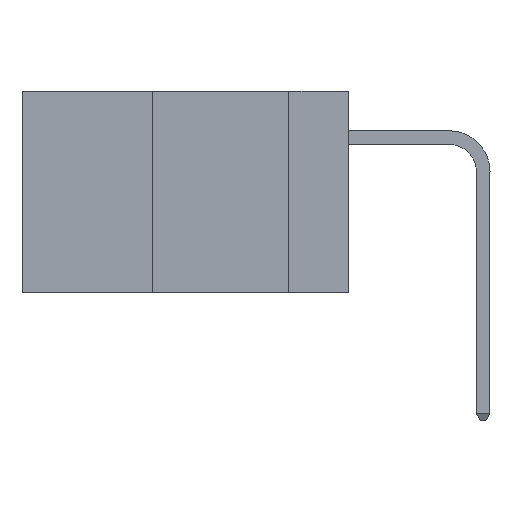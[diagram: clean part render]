
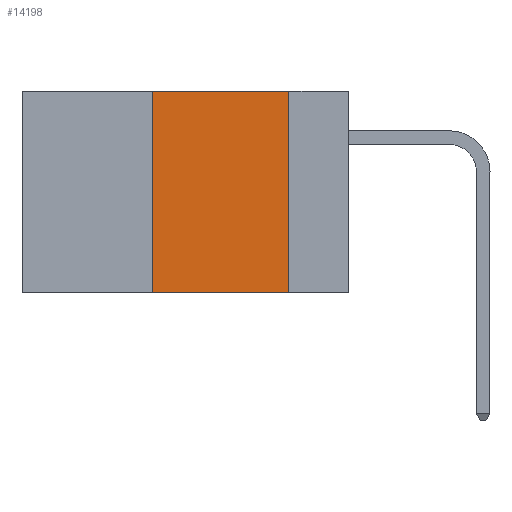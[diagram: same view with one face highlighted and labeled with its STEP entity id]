
A CAD part, left-side view. The second image highlights one B-rep face of the part: STEP entity #14198.
In plain terms, the highlighted planar face has unit normal (-1, 0, 0).
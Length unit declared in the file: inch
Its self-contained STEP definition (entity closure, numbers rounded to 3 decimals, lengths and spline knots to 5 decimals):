
#286 = LINE ( 'NONE', #26211, #30378 ) ;
#322 = ORIENTED_EDGE ( 'NONE', *, *, #28222, .F. ) ;
#530 = DIRECTION ( 'NONE',  ( 0., -1., 0. ) ) ;
#1850 = ORIENTED_EDGE ( 'NONE', *, *, #7102, .T. ) ;
#1885 = LINE ( 'NONE', #28804, #24264 ) ;
#4519 = EDGE_CURVE ( 'NONE', #36708, #11332, #286, .T. ) ;
#5098 = VECTOR ( 'NONE', #530, 39.37008 ) ;
#7102 = EDGE_CURVE ( 'NONE', #7261, #11332, #21603, .T. ) ;
#7261 = VERTEX_POINT ( 'NONE', #18776 ) ;
#9063 = PLANE ( 'NONE',  #30794 ) ;
#10246 = VERTEX_POINT ( 'NONE', #14431 ) ;
#11332 = VERTEX_POINT ( 'NONE', #33572 ) ;
#11418 = EDGE_LOOP ( 'NONE', ( #18640, #14074, #322, #1850 ) ) ;
#12031 = DIRECTION ( 'NONE',  ( 1., 0., 0. ) ) ;
#13965 = FACE_OUTER_BOUND ( 'NONE', #11418, .T. ) ;
#14074 = ORIENTED_EDGE ( 'NONE', *, *, #23675, .F. ) ;
#14198 = ADVANCED_FACE ( 'NONE', ( #13965 ), #9063, .F. ) ;
#14431 = CARTESIAN_POINT ( 'NONE',  ( 0., 0.36, 0. ) ) ;
#16020 = CARTESIAN_POINT ( 'NONE',  ( 0., 0.11, 0. ) ) ;
#18135 = CARTESIAN_POINT ( 'NONE',  ( 0., 0.6, -0.37 ) ) ;
#18640 = ORIENTED_EDGE ( 'NONE', *, *, #4519, .F. ) ;
#18776 = CARTESIAN_POINT ( 'NONE',  ( 0., 0.36, -0.37 ) ) ;
#20173 = VECTOR ( 'NONE', #25773, 39.37008 ) ;
#20572 = DIRECTION ( 'NONE',  ( 0., 0., -1. ) ) ;
#21603 = LINE ( 'NONE', #18135, #5098 ) ;
#22890 = CARTESIAN_POINT ( 'NONE',  ( 0., 0.6, 0. ) ) ;
#23675 = EDGE_CURVE ( 'NONE', #10246, #36708, #27820, .T. ) ;
#24264 = VECTOR ( 'NONE', #26007, 39.37008 ) ;
#25773 = DIRECTION ( 'NONE',  ( 0., -1., 0. ) ) ;
#26007 = DIRECTION ( 'NONE',  ( 0., 0., 1. ) ) ;
#26211 = CARTESIAN_POINT ( 'NONE',  ( 0., 0.11, 0. ) ) ;
#27820 = LINE ( 'NONE', #22890, #20173 ) ;
#28222 = EDGE_CURVE ( 'NONE', #7261, #10246, #1885, .T. ) ;
#28804 = CARTESIAN_POINT ( 'NONE',  ( 0., 0.36, 0. ) ) ;
#29323 = CARTESIAN_POINT ( 'NONE',  ( 0., 0.6, 0. ) ) ;
#30378 = VECTOR ( 'NONE', #20572, 39.37008 ) ;
#30794 = AXIS2_PLACEMENT_3D ( 'NONE', #29323, #12031, #32176 ) ;
#32176 = DIRECTION ( 'NONE',  ( 0., 0., -1. ) ) ;
#33572 = CARTESIAN_POINT ( 'NONE',  ( 0., 0.11, -0.37 ) ) ;
#36708 = VERTEX_POINT ( 'NONE', #16020 ) ;
